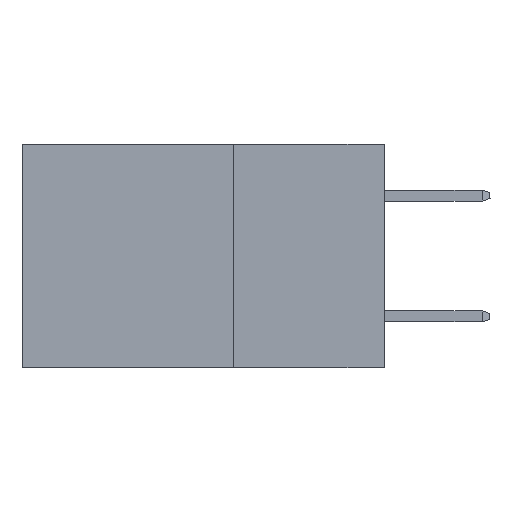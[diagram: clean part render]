
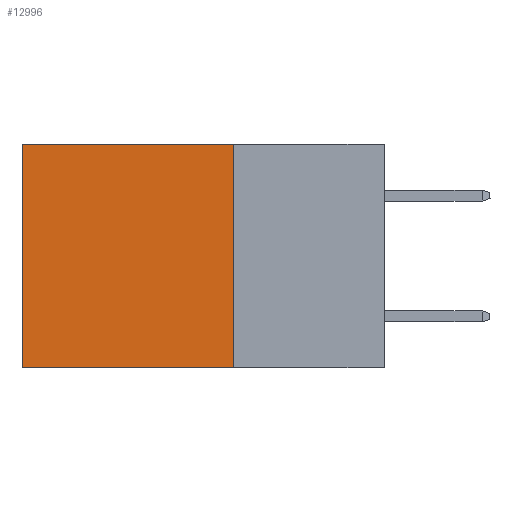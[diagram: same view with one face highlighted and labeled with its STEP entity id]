
A CAD part, left-side view. The second image highlights one B-rep face of the part: STEP entity #12996.
In plain terms, the highlighted planar face has unit normal (-1, 0, 0).
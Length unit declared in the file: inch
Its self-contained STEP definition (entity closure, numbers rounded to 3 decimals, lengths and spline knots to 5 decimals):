
#90 = CARTESIAN_POINT ( 'NONE',  ( 0.298, 0.6, 0. ) ) ;
#268 = CARTESIAN_POINT ( 'NONE',  ( 0.298, 0.25, 0. ) ) ;
#1325 = DIRECTION ( 'NONE',  ( 1., 0., 0. ) ) ;
#2060 = VECTOR ( 'NONE', #18449, 39.37008 ) ;
#2384 = LINE ( 'NONE', #9851, #9960 ) ;
#4258 = VECTOR ( 'NONE', #11683, 39.37008 ) ;
#4475 = ORIENTED_EDGE ( 'NONE', *, *, #17274, .T. ) ;
#4903 = ORIENTED_EDGE ( 'NONE', *, *, #11793, .F. ) ;
#5177 = LINE ( 'NONE', #20234, #20562 ) ;
#7613 = CARTESIAN_POINT ( 'NONE',  ( 0.298, 0.25, -0.37 ) ) ;
#7633 = CARTESIAN_POINT ( 'NONE',  ( 0.298, 0.6, -0.37 ) ) ;
#9357 = VERTEX_POINT ( 'NONE', #90 ) ;
#9473 = DIRECTION ( 'NONE',  ( 0., 0., -1. ) ) ;
#9851 = CARTESIAN_POINT ( 'NONE',  ( 0.298, 0.6, 0. ) ) ;
#9960 = VECTOR ( 'NONE', #21884, 39.37008 ) ;
#11163 = AXIS2_PLACEMENT_3D ( 'NONE', #19503, #1325, #9473 ) ;
#11683 = DIRECTION ( 'NONE',  ( 0., 1., 0. ) ) ;
#11793 = EDGE_CURVE ( 'NONE', #24068, #17596, #15659, .T. ) ;
#12820 = LINE ( 'NONE', #268, #2060 ) ;
#12996 = ADVANCED_FACE ( 'NONE', ( #23409 ), #21516, .F. ) ;
#13203 = ORIENTED_EDGE ( 'NONE', *, *, #19106, .F. ) ;
#14174 = ORIENTED_EDGE ( 'NONE', *, *, #17053, .T. ) ;
#14309 = DIRECTION ( 'NONE',  ( 0., 0., -1. ) ) ;
#15659 = LINE ( 'NONE', #7613, #4258 ) ;
#15858 = CARTESIAN_POINT ( 'NONE',  ( 0.298, 0.25, -0.37 ) ) ;
#16095 = VERTEX_POINT ( 'NONE', #16946 ) ;
#16946 = CARTESIAN_POINT ( 'NONE',  ( 0.298, 0.25, 0. ) ) ;
#17053 = EDGE_CURVE ( 'NONE', #9357, #17596, #2384, .T. ) ;
#17274 = EDGE_CURVE ( 'NONE', #16095, #9357, #12820, .T. ) ;
#17596 = VERTEX_POINT ( 'NONE', #7633 ) ;
#18449 = DIRECTION ( 'NONE',  ( 0., 1., 0. ) ) ;
#19106 = EDGE_CURVE ( 'NONE', #16095, #24068, #5177, .T. ) ;
#19503 = CARTESIAN_POINT ( 'NONE',  ( 0.298, 0.25, 0. ) ) ;
#20234 = CARTESIAN_POINT ( 'NONE',  ( 0.298, 0.25, 0. ) ) ;
#20562 = VECTOR ( 'NONE', #14309, 39.37008 ) ;
#21516 = PLANE ( 'NONE',  #11163 ) ;
#21884 = DIRECTION ( 'NONE',  ( 0., 0., -1. ) ) ;
#23153 = EDGE_LOOP ( 'NONE', ( #14174, #4903, #13203, #4475 ) ) ;
#23409 = FACE_OUTER_BOUND ( 'NONE', #23153, .T. ) ;
#24068 = VERTEX_POINT ( 'NONE', #15858 ) ;
